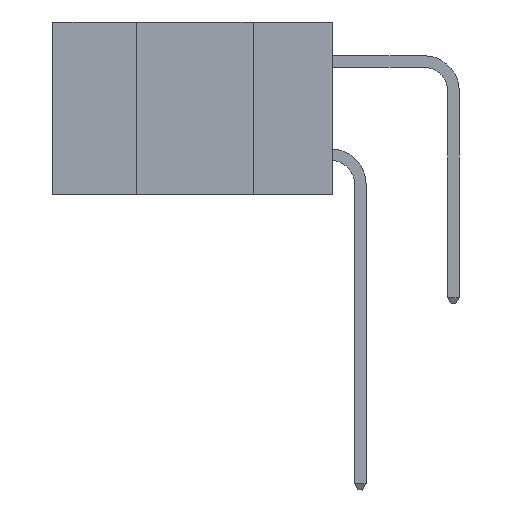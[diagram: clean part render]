
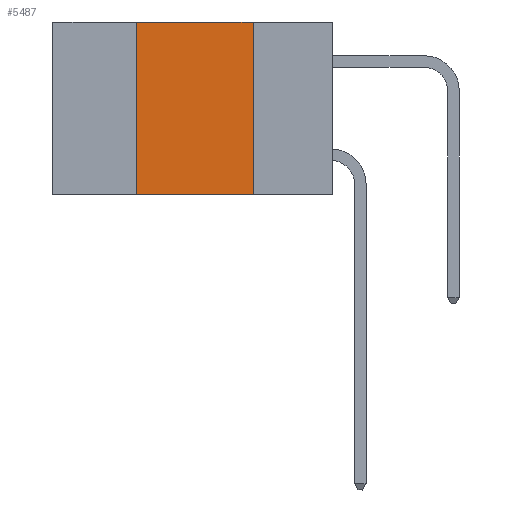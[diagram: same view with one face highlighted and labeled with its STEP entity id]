
A CAD part, left-side view. The second image highlights one B-rep face of the part: STEP entity #5487.
In plain terms, the highlighted planar face has unit normal (-1, 0, 0).
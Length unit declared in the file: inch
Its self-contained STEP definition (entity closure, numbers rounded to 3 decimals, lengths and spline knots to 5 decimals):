
#183 = VECTOR ( 'NONE', #9040, 39.37008 ) ;
#297 = EDGE_CURVE ( 'NONE', #1779, #2697, #10149, .T. ) ;
#1094 = VECTOR ( 'NONE', #3672, 39.37008 ) ;
#1779 = VERTEX_POINT ( 'NONE', #8339 ) ;
#2525 = LINE ( 'NONE', #6398, #1094 ) ;
#2697 = VERTEX_POINT ( 'NONE', #10007 ) ;
#3221 = CARTESIAN_POINT ( 'NONE',  ( 0., 0.17, -0.37 ) ) ;
#3672 = DIRECTION ( 'NONE',  ( 0., -1., 0. ) ) ;
#3827 = EDGE_CURVE ( 'NONE', #2697, #5498, #2525, .T. ) ;
#5200 = DIRECTION ( 'NONE',  ( 0., 0., 1. ) ) ;
#5487 = ADVANCED_FACE ( 'NONE', ( #7038 ), #10735, .F. ) ;
#5498 = VERTEX_POINT ( 'NONE', #11044 ) ;
#5921 = LINE ( 'NONE', #11495, #11852 ) ;
#6116 = CARTESIAN_POINT ( 'NONE',  ( 0., 0.6, 0. ) ) ;
#6356 = ORIENTED_EDGE ( 'NONE', *, *, #297, .F. ) ;
#6398 = CARTESIAN_POINT ( 'NONE',  ( 0., 0.6, 0. ) ) ;
#6580 = EDGE_CURVE ( 'NONE', #5498, #11264, #7988, .T. ) ;
#6617 = DIRECTION ( 'NONE',  ( 1., 0., 0. ) ) ;
#7038 = FACE_OUTER_BOUND ( 'NONE', #7722, .T. ) ;
#7722 = EDGE_LOOP ( 'NONE', ( #8691, #11331, #6356, #9876 ) ) ;
#7988 = LINE ( 'NONE', #10962, #183 ) ;
#8339 = CARTESIAN_POINT ( 'NONE',  ( 0., 0.42, -0.37 ) ) ;
#8691 = ORIENTED_EDGE ( 'NONE', *, *, #6580, .F. ) ;
#8736 = DIRECTION ( 'NONE',  ( 0., -1., 0. ) ) ;
#8843 = EDGE_CURVE ( 'NONE', #1779, #11264, #5921, .T. ) ;
#9040 = DIRECTION ( 'NONE',  ( 0., 0., -1. ) ) ;
#9837 = DIRECTION ( 'NONE',  ( 0., 0., -1. ) ) ;
#9876 = ORIENTED_EDGE ( 'NONE', *, *, #8843, .T. ) ;
#10007 = CARTESIAN_POINT ( 'NONE',  ( 0., 0.42, 0. ) ) ;
#10149 = LINE ( 'NONE', #11815, #10930 ) ;
#10735 = PLANE ( 'NONE',  #10831 ) ;
#10831 = AXIS2_PLACEMENT_3D ( 'NONE', #6116, #6617, #9837 ) ;
#10930 = VECTOR ( 'NONE', #5200, 39.37008 ) ;
#10962 = CARTESIAN_POINT ( 'NONE',  ( 0., 0.17, -0.37 ) ) ;
#11044 = CARTESIAN_POINT ( 'NONE',  ( 0., 0.17, 0. ) ) ;
#11264 = VERTEX_POINT ( 'NONE', #3221 ) ;
#11331 = ORIENTED_EDGE ( 'NONE', *, *, #3827, .F. ) ;
#11495 = CARTESIAN_POINT ( 'NONE',  ( 0., 0.6, -0.37 ) ) ;
#11815 = CARTESIAN_POINT ( 'NONE',  ( 0., 0.42, -0.37 ) ) ;
#11852 = VECTOR ( 'NONE', #8736, 39.37008 ) ;
